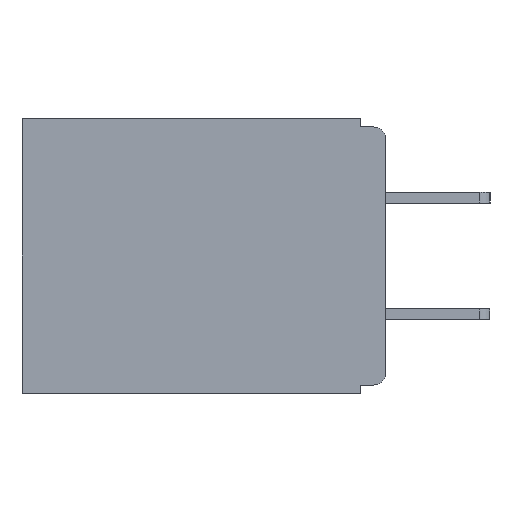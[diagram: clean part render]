
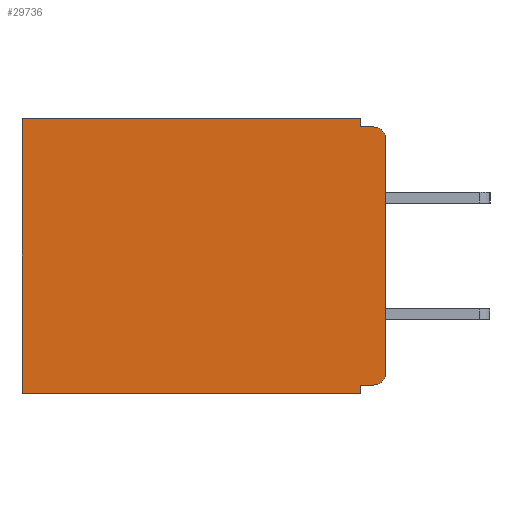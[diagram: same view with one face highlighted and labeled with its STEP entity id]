
A CAD part, left-side view. The second image highlights one B-rep face of the part: STEP entity #29736.
In plain terms, the highlighted planar face has unit normal (-1, 0, 0).
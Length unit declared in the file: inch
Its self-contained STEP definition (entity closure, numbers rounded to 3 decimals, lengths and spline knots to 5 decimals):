
#815 = ORIENTED_EDGE ( 'NONE', *, *, #22362, .T. ) ;
#826 = AXIS2_PLACEMENT_3D ( 'NONE', #22585, #7643, #25086 ) ;
#1104 = LINE ( 'NONE', #10237, #19415 ) ;
#1466 = VECTOR ( 'NONE', #25265, 39.37008 ) ;
#1754 = VERTEX_POINT ( 'NONE', #25470 ) ;
#2178 = LINE ( 'NONE', #23546, #21295 ) ;
#3052 = LINE ( 'NONE', #32068, #10460 ) ;
#3345 = CIRCLE ( 'NONE', #826, 0.015 ) ;
#3420 = DIRECTION ( 'NONE',  ( 0., 1., 0. ) ) ;
#5353 = DIRECTION ( 'NONE',  ( 0., 0., -1. ) ) ;
#5691 = VERTEX_POINT ( 'NONE', #29315 ) ;
#6799 = CARTESIAN_POINT ( 'NONE',  ( 0.3, 0.031, 0. ) ) ;
#6953 = VERTEX_POINT ( 'NONE', #19217 ) ;
#6956 = VERTEX_POINT ( 'NONE', #6799 ) ;
#7643 = DIRECTION ( 'NONE',  ( -1., 0., 0. ) ) ;
#8210 = EDGE_CURVE ( 'NONE', #6956, #6953, #3052, .T. ) ;
#8243 = CIRCLE ( 'NONE', #18571, 0.015 ) ;
#8689 = CARTESIAN_POINT ( 'NONE',  ( 0.3, 0.437, -0.33 ) ) ;
#9017 = EDGE_CURVE ( 'NONE', #6953, #18684, #28161, .T. ) ;
#9424 = CARTESIAN_POINT ( 'NONE',  ( 0.3, 0.031, 0. ) ) ;
#9439 = ORIENTED_EDGE ( 'NONE', *, *, #30683, .F. ) ;
#10237 = CARTESIAN_POINT ( 'NONE',  ( 0.3, 0., -0.01 ) ) ;
#10344 = DIRECTION ( 'NONE',  ( 0., -1., 0. ) ) ;
#10460 = VECTOR ( 'NONE', #17187, 39.37008 ) ;
#11028 = ORIENTED_EDGE ( 'NONE', *, *, #27820, .F. ) ;
#11675 = EDGE_CURVE ( 'NONE', #27811, #18684, #20566, .T. ) ;
#11948 = ORIENTED_EDGE ( 'NONE', *, *, #8210, .T. ) ;
#12099 = PLANE ( 'NONE',  #28746 ) ;
#12210 = DIRECTION ( 'NONE',  ( 0., 0., -1. ) ) ;
#12338 = CARTESIAN_POINT ( 'NONE',  ( 0.3, 0.031, -0.32 ) ) ;
#12344 = EDGE_CURVE ( 'NONE', #24059, #25030, #3345, .T. ) ;
#12580 = EDGE_CURVE ( 'NONE', #20289, #27811, #2178, .T. ) ;
#12862 = DIRECTION ( 'NONE',  ( 0., 0., -1. ) ) ;
#13516 = DIRECTION ( 'NONE',  ( -1., 0., 0. ) ) ;
#13778 = ORIENTED_EDGE ( 'NONE', *, *, #25092, .F. ) ;
#13875 = LINE ( 'NONE', #9424, #19725 ) ;
#14413 = DIRECTION ( 'NONE',  ( 0., 0., -1. ) ) ;
#14850 = VECTOR ( 'NONE', #12862, 39.37008 ) ;
#15187 = ORIENTED_EDGE ( 'NONE', *, *, #12580, .F. ) ;
#15238 = CARTESIAN_POINT ( 'NONE',  ( 0.3, 0.031, -0.33 ) ) ;
#15469 = ORIENTED_EDGE ( 'NONE', *, *, #9017, .T. ) ;
#17187 = DIRECTION ( 'NONE',  ( 0., 1., 0. ) ) ;
#17222 = ORIENTED_EDGE ( 'NONE', *, *, #12344, .T. ) ;
#17384 = CARTESIAN_POINT ( 'NONE',  ( 0.3, 0., -0.33 ) ) ;
#17591 = EDGE_CURVE ( 'NONE', #6956, #5691, #13875, .T. ) ;
#18241 = CARTESIAN_POINT ( 'NONE',  ( 0.3, 0., -0.025 ) ) ;
#18571 = AXIS2_PLACEMENT_3D ( 'NONE', #28454, #13516, #30907 ) ;
#18658 = VECTOR ( 'NONE', #3420, 39.37008 ) ;
#18684 = VERTEX_POINT ( 'NONE', #8689 ) ;
#19217 = CARTESIAN_POINT ( 'NONE',  ( 0.3, 0.437, 0. ) ) ;
#19415 = VECTOR ( 'NONE', #10344, 39.37008 ) ;
#19725 = VECTOR ( 'NONE', #14413, 39.37008 ) ;
#20289 = VERTEX_POINT ( 'NONE', #12338 ) ;
#20303 = CARTESIAN_POINT ( 'NONE',  ( 0.3, 0., -0.33 ) ) ;
#20566 = LINE ( 'NONE', #17384, #1466 ) ;
#20996 = ORIENTED_EDGE ( 'NONE', *, *, #11675, .F. ) ;
#21295 = VECTOR ( 'NONE', #26064, 39.37008 ) ;
#22362 = EDGE_CURVE ( 'NONE', #27299, #1754, #8243, .T. ) ;
#22585 = CARTESIAN_POINT ( 'NONE',  ( 0.3, 0.015, -0.305 ) ) ;
#23546 = CARTESIAN_POINT ( 'NONE',  ( 0.3, 0.031, -0.33 ) ) ;
#24059 = VERTEX_POINT ( 'NONE', #25794 ) ;
#24637 = CARTESIAN_POINT ( 'NONE',  ( 0.3, 0., -0.33 ) ) ;
#25030 = VERTEX_POINT ( 'NONE', #27579 ) ;
#25086 = DIRECTION ( 'NONE',  ( 0., 0., -1. ) ) ;
#25092 = EDGE_CURVE ( 'NONE', #5691, #1754, #1104, .T. ) ;
#25265 = DIRECTION ( 'NONE',  ( 0., 1., 0. ) ) ;
#25307 = LINE ( 'NONE', #30750, #18658 ) ;
#25470 = CARTESIAN_POINT ( 'NONE',  ( 0.3, 0.015, -0.01 ) ) ;
#25520 = ORIENTED_EDGE ( 'NONE', *, *, #17591, .F. ) ;
#25794 = CARTESIAN_POINT ( 'NONE',  ( 0.3, 0.015, -0.32 ) ) ;
#26064 = DIRECTION ( 'NONE',  ( 0., 0., -1. ) ) ;
#27034 = VECTOR ( 'NONE', #5353, 39.37008 ) ;
#27155 = DIRECTION ( 'NONE',  ( 1., 0., 0. ) ) ;
#27284 = FACE_OUTER_BOUND ( 'NONE', #29187, .T. ) ;
#27299 = VERTEX_POINT ( 'NONE', #18241 ) ;
#27579 = CARTESIAN_POINT ( 'NONE',  ( 0.3, 0., -0.305 ) ) ;
#27811 = VERTEX_POINT ( 'NONE', #15238 ) ;
#27820 = EDGE_CURVE ( 'NONE', #27299, #25030, #32025, .T. ) ;
#28161 = LINE ( 'NONE', #30382, #14850 ) ;
#28454 = CARTESIAN_POINT ( 'NONE',  ( 0.3, 0.015, -0.025 ) ) ;
#28746 = AXIS2_PLACEMENT_3D ( 'NONE', #24637, #27155, #12210 ) ;
#29187 = EDGE_LOOP ( 'NONE', ( #11028, #815, #13778, #25520, #11948, #15469, #20996, #15187, #9439, #17222 ) ) ;
#29315 = CARTESIAN_POINT ( 'NONE',  ( 0.3, 0.031, -0.01 ) ) ;
#29736 = ADVANCED_FACE ( 'NONE', ( #27284 ), #12099, .F. ) ;
#30382 = CARTESIAN_POINT ( 'NONE',  ( 0.3, 0.437, -0.33 ) ) ;
#30683 = EDGE_CURVE ( 'NONE', #24059, #20289, #25307, .T. ) ;
#30750 = CARTESIAN_POINT ( 'NONE',  ( 0.3, 0., -0.32 ) ) ;
#30907 = DIRECTION ( 'NONE',  ( 0., 0., -1. ) ) ;
#32025 = LINE ( 'NONE', #20303, #27034 ) ;
#32068 = CARTESIAN_POINT ( 'NONE',  ( 0.3, 0., 0. ) ) ;
